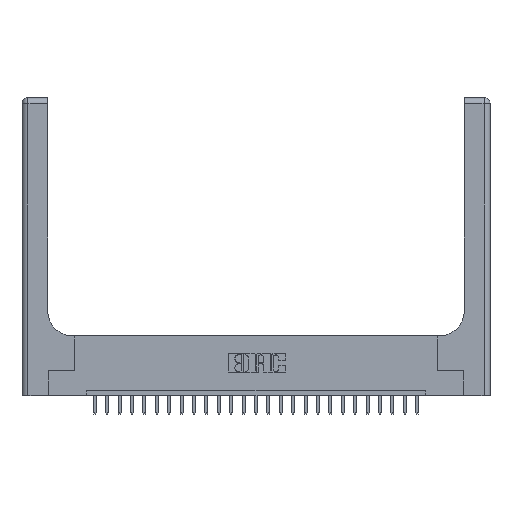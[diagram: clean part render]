
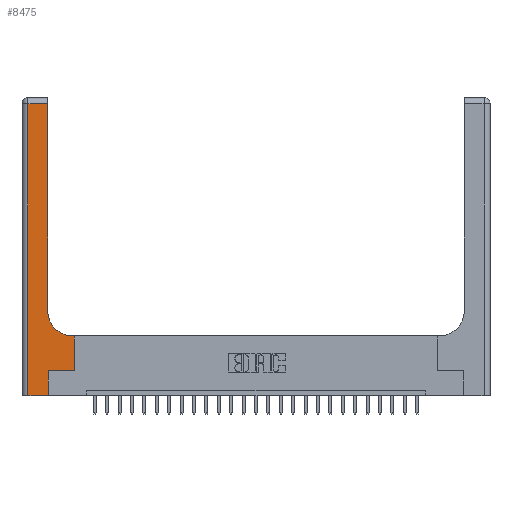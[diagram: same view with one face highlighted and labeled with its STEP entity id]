
A CAD part, top view. The second image highlights one B-rep face of the part: STEP entity #8475.
In plain terms, the highlighted planar face has unit normal (0, 0, 1).
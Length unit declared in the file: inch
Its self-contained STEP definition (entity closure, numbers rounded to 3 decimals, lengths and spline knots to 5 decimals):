
#18 = EDGE_CURVE ( 'NONE', #2295, #4385, #8976, .T. ) ;
#415 = CIRCLE ( 'NONE', #9217, 0.25 ) ;
#657 = CARTESIAN_POINT ( 'NONE',  ( 0.528, 0.25, 0.37 ) ) ;
#1581 = LINE ( 'NONE', #18766, #12405 ) ;
#2292 = DIRECTION ( 'NONE',  ( -1., 0., 0. ) ) ;
#2295 = VERTEX_POINT ( 'NONE', #20904 ) ;
#2378 = LINE ( 'NONE', #22206, #16100 ) ;
#2424 = EDGE_CURVE ( 'NONE', #12832, #2295, #1581, .T. ) ;
#2593 = EDGE_CURVE ( 'NONE', #10008, #3421, #415, .T. ) ;
#2787 = CARTESIAN_POINT ( 'NONE',  ( 0.528, 0.6, 0.37 ) ) ;
#3421 = VERTEX_POINT ( 'NONE', #9825 ) ;
#3464 = VECTOR ( 'NONE', #11454, 39.37008 ) ;
#3679 = DIRECTION ( 'NONE',  ( 1., 0., 0. ) ) ;
#3936 = EDGE_CURVE ( 'NONE', #3421, #22701, #2378, .T. ) ;
#3945 = DIRECTION ( 'NONE',  ( 0., 1., 0. ) ) ;
#4289 = CARTESIAN_POINT ( 'NONE',  ( 0., 2.94, 0.37 ) ) ;
#4385 = VERTEX_POINT ( 'NONE', #21654 ) ;
#4813 = CARTESIAN_POINT ( 'NONE',  ( 0.51, 0.85, 0.37 ) ) ;
#4828 = VECTOR ( 'NONE', #23915, 39.37008 ) ;
#5884 = ORIENTED_EDGE ( 'NONE', *, *, #18, .T. ) ;
#6044 = EDGE_CURVE ( 'NONE', #4385, #8482, #23381, .T. ) ;
#6484 = ORIENTED_EDGE ( 'NONE', *, *, #15334, .T. ) ;
#6551 = ORIENTED_EDGE ( 'NONE', *, *, #6044, .T. ) ;
#6552 = CARTESIAN_POINT ( 'NONE',  ( 0.265, 0., 0.37 ) ) ;
#7197 = CARTESIAN_POINT ( 'NONE',  ( 0.265, 0.25, 0.37 ) ) ;
#7309 = LINE ( 'NONE', #657, #21528 ) ;
#7316 = CARTESIAN_POINT ( 'NONE',  ( 0.06, 0., 0.37 ) ) ;
#7743 = DIRECTION ( 'NONE',  ( -1., 0., 0. ) ) ;
#8475 = ADVANCED_FACE ( 'NONE', ( #9653 ), #11370, .F. ) ;
#8482 = VERTEX_POINT ( 'NONE', #9402 ) ;
#8976 = LINE ( 'NONE', #6552, #21758 ) ;
#9217 = AXIS2_PLACEMENT_3D ( 'NONE', #4813, #10316, #13737 ) ;
#9402 = CARTESIAN_POINT ( 'NONE',  ( 0.528, 0.25, 0.37 ) ) ;
#9653 = FACE_OUTER_BOUND ( 'NONE', #10556, .T. ) ;
#9730 = EDGE_CURVE ( 'NONE', #19595, #10008, #20029, .T. ) ;
#9825 = CARTESIAN_POINT ( 'NONE',  ( 0.26, 0.85, 0.37 ) ) ;
#10008 = VERTEX_POINT ( 'NONE', #22518 ) ;
#10021 = DIRECTION ( 'NONE',  ( 0., 1., 0. ) ) ;
#10046 = VERTEX_POINT ( 'NONE', #19261 ) ;
#10316 = DIRECTION ( 'NONE',  ( 0., 0., -1. ) ) ;
#10556 = EDGE_LOOP ( 'NONE', ( #21006, #6484, #11954, #17414, #5884, #6551, #21053, #22092, #19272 ) ) ;
#11182 = LINE ( 'NONE', #4289, #22188 ) ;
#11370 = PLANE ( 'NONE',  #21386 ) ;
#11454 = DIRECTION ( 'NONE',  ( -1., 0., 0. ) ) ;
#11954 = ORIENTED_EDGE ( 'NONE', *, *, #21115, .T. ) ;
#12118 = VECTOR ( 'NONE', #13068, 39.37008 ) ;
#12405 = VECTOR ( 'NONE', #3679, 39.37008 ) ;
#12703 = DIRECTION ( 'NONE',  ( 0., 1., 0. ) ) ;
#12832 = VERTEX_POINT ( 'NONE', #7316 ) ;
#13068 = DIRECTION ( 'NONE',  ( 0., -1., 0. ) ) ;
#13737 = DIRECTION ( 'NONE',  ( 1., 0., 0. ) ) ;
#14766 = CARTESIAN_POINT ( 'NONE',  ( 0.06, 3., 0.37 ) ) ;
#15334 = EDGE_CURVE ( 'NONE', #22701, #10046, #11182, .T. ) ;
#16100 = VECTOR ( 'NONE', #3945, 39.37008 ) ;
#16354 = CARTESIAN_POINT ( 'NONE',  ( 0.26, 2.94, 0.37 ) ) ;
#16524 = EDGE_CURVE ( 'NONE', #8482, #19595, #7309, .T. ) ;
#16712 = CARTESIAN_POINT ( 'NONE',  ( 0., 3., 0.37 ) ) ;
#17414 = ORIENTED_EDGE ( 'NONE', *, *, #2424, .T. ) ;
#18563 = CARTESIAN_POINT ( 'NONE',  ( 0.26, 0.6, 0.37 ) ) ;
#18766 = CARTESIAN_POINT ( 'NONE',  ( 0., 0., 0.37 ) ) ;
#18885 = DIRECTION ( 'NONE',  ( 0., 0., -1. ) ) ;
#19261 = CARTESIAN_POINT ( 'NONE',  ( 0.06, 2.94, 0.37 ) ) ;
#19272 = ORIENTED_EDGE ( 'NONE', *, *, #2593, .T. ) ;
#19595 = VERTEX_POINT ( 'NONE', #2787 ) ;
#20029 = LINE ( 'NONE', #18563, #3464 ) ;
#20904 = CARTESIAN_POINT ( 'NONE',  ( 0.265, 0., 0.37 ) ) ;
#21006 = ORIENTED_EDGE ( 'NONE', *, *, #3936, .T. ) ;
#21053 = ORIENTED_EDGE ( 'NONE', *, *, #16524, .T. ) ;
#21115 = EDGE_CURVE ( 'NONE', #10046, #12832, #23706, .T. ) ;
#21386 = AXIS2_PLACEMENT_3D ( 'NONE', #16712, #18885, #7743 ) ;
#21528 = VECTOR ( 'NONE', #10021, 39.37008 ) ;
#21654 = CARTESIAN_POINT ( 'NONE',  ( 0.265, 0.25, 0.37 ) ) ;
#21758 = VECTOR ( 'NONE', #12703, 39.37008 ) ;
#22092 = ORIENTED_EDGE ( 'NONE', *, *, #9730, .T. ) ;
#22188 = VECTOR ( 'NONE', #2292, 39.37008 ) ;
#22206 = CARTESIAN_POINT ( 'NONE',  ( 0.26, 3., 0.37 ) ) ;
#22518 = CARTESIAN_POINT ( 'NONE',  ( 0.51, 0.6, 0.37 ) ) ;
#22701 = VERTEX_POINT ( 'NONE', #16354 ) ;
#23381 = LINE ( 'NONE', #7197, #4828 ) ;
#23706 = LINE ( 'NONE', #14766, #12118 ) ;
#23915 = DIRECTION ( 'NONE',  ( 1., 0., 0. ) ) ;
